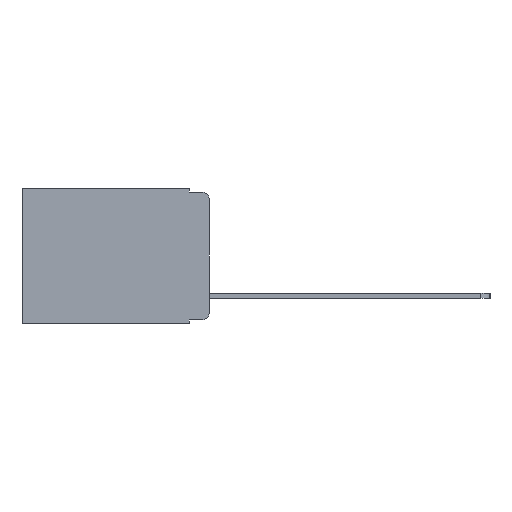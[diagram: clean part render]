
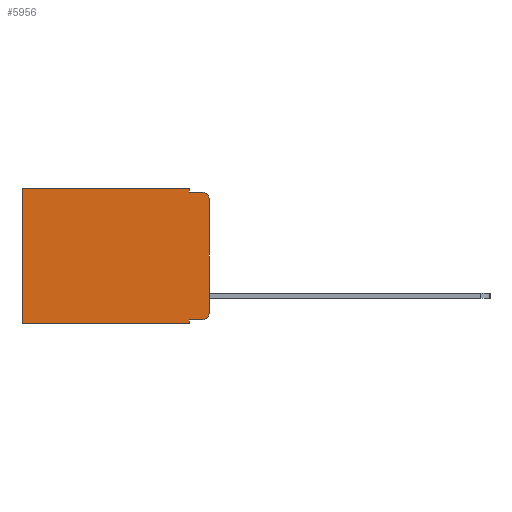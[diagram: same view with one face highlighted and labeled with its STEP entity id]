
A CAD part, left-side view. The second image highlights one B-rep face of the part: STEP entity #5956.
In plain terms, the highlighted planar face has unit normal (-1, 0, 0).
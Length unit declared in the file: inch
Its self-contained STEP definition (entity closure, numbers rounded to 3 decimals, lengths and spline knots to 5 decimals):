
#191 = DIRECTION ( 'NONE',  ( 0., 0., -1. ) ) ;
#523 = CARTESIAN_POINT ( 'NONE',  ( 0.298, 0.051, 0. ) ) ;
#1885 = VERTEX_POINT ( 'NONE', #18534 ) ;
#2325 = VERTEX_POINT ( 'NONE', #20795 ) ;
#2650 = CARTESIAN_POINT ( 'NONE',  ( 0.298, 0.051, -0.01 ) ) ;
#2840 = ORIENTED_EDGE ( 'NONE', *, *, #15150, .T. ) ;
#3032 = DIRECTION ( 'NONE',  ( 0., 1., 0. ) ) ;
#3076 = EDGE_CURVE ( 'NONE', #10299, #19480, #10213, .T. ) ;
#3449 = CARTESIAN_POINT ( 'NONE',  ( 0.298, 0., -0.03 ) ) ;
#4830 = DIRECTION ( 'NONE',  ( 0., 0., -1. ) ) ;
#4920 = EDGE_CURVE ( 'NONE', #17954, #14853, #17145, .T. ) ;
#5129 = VECTOR ( 'NONE', #13450, 39.37008 ) ;
#5503 = AXIS2_PLACEMENT_3D ( 'NONE', #19435, #8144, #21201 ) ;
#5956 = ADVANCED_FACE ( 'NONE', ( #15902 ), #20668, .F. ) ;
#6232 = EDGE_CURVE ( 'NONE', #10166, #14853, #13845, .T. ) ;
#6737 = VECTOR ( 'NONE', #15516, 39.37008 ) ;
#7213 = ORIENTED_EDGE ( 'NONE', *, *, #18138, .F. ) ;
#7403 = ORIENTED_EDGE ( 'NONE', *, *, #11337, .F. ) ;
#7589 = CARTESIAN_POINT ( 'NONE',  ( 0.298, 0., 0. ) ) ;
#7990 = ORIENTED_EDGE ( 'NONE', *, *, #10050, .T. ) ;
#8144 = DIRECTION ( 'NONE',  ( -1., 0., 0. ) ) ;
#8494 = ORIENTED_EDGE ( 'NONE', *, *, #6232, .F. ) ;
#8585 = ORIENTED_EDGE ( 'NONE', *, *, #8775, .F. ) ;
#8637 = CARTESIAN_POINT ( 'NONE',  ( 0.298, 0.473, -0.343 ) ) ;
#8775 = EDGE_CURVE ( 'NONE', #10299, #10166, #18687, .T. ) ;
#9145 = VERTEX_POINT ( 'NONE', #8637 ) ;
#9196 = EDGE_LOOP ( 'NONE', ( #7213, #16076, #8494, #8585, #18636, #7990, #13047, #7403, #2840, #11280 ) ) ;
#9250 = VECTOR ( 'NONE', #4830, 39.37008 ) ;
#9460 = DIRECTION ( 'NONE',  ( 1., 0., 0. ) ) ;
#9505 = CARTESIAN_POINT ( 'NONE',  ( 0.298, 0.02, -0.03 ) ) ;
#9752 = VECTOR ( 'NONE', #20684, 39.37008 ) ;
#10050 = EDGE_CURVE ( 'NONE', #19480, #9145, #14839, .T. ) ;
#10166 = VERTEX_POINT ( 'NONE', #17454 ) ;
#10213 = LINE ( 'NONE', #22612, #5129 ) ;
#10299 = VERTEX_POINT ( 'NONE', #523 ) ;
#10705 = CARTESIAN_POINT ( 'NONE',  ( 0.298, 0., -0.343 ) ) ;
#11264 = AXIS2_PLACEMENT_3D ( 'NONE', #9505, #22533, #11455 ) ;
#11280 = ORIENTED_EDGE ( 'NONE', *, *, #16379, .T. ) ;
#11334 = CARTESIAN_POINT ( 'NONE',  ( 0.298, 0.051, 0. ) ) ;
#11337 = EDGE_CURVE ( 'NONE', #19184, #1885, #24091, .T. ) ;
#11455 = DIRECTION ( 'NONE',  ( 0., 0., -1. ) ) ;
#11761 = CARTESIAN_POINT ( 'NONE',  ( 0.298, 0., 0. ) ) ;
#12386 = LINE ( 'NONE', #13709, #6737 ) ;
#12438 = CARTESIAN_POINT ( 'NONE',  ( 0.298, 0.051, 0. ) ) ;
#12877 = LINE ( 'NONE', #10705, #17303 ) ;
#13047 = ORIENTED_EDGE ( 'NONE', *, *, #17810, .F. ) ;
#13450 = DIRECTION ( 'NONE',  ( 0., 1., 0. ) ) ;
#13705 = VECTOR ( 'NONE', #18805, 39.37008 ) ;
#13709 = CARTESIAN_POINT ( 'NONE',  ( 0.298, 0.051, -0.333 ) ) ;
#13845 = LINE ( 'NONE', #2650, #18266 ) ;
#14839 = LINE ( 'NONE', #17037, #9752 ) ;
#14853 = VERTEX_POINT ( 'NONE', #22093 ) ;
#15150 = EDGE_CURVE ( 'NONE', #19184, #2325, #12386, .T. ) ;
#15516 = DIRECTION ( 'NONE',  ( 0., -1., 0. ) ) ;
#15902 = FACE_OUTER_BOUND ( 'NONE', #9196, .T. ) ;
#16076 = ORIENTED_EDGE ( 'NONE', *, *, #4920, .T. ) ;
#16379 = EDGE_CURVE ( 'NONE', #2325, #23035, #20991, .T. ) ;
#17037 = CARTESIAN_POINT ( 'NONE',  ( 0.298, 0.473, 0. ) ) ;
#17145 = CIRCLE ( 'NONE', #11264, 0.02 ) ;
#17303 = VECTOR ( 'NONE', #3032, 39.37008 ) ;
#17454 = CARTESIAN_POINT ( 'NONE',  ( 0.298, 0.051, -0.01 ) ) ;
#17810 = EDGE_CURVE ( 'NONE', #1885, #9145, #12877, .T. ) ;
#17922 = DIRECTION ( 'NONE',  ( 0., -1., 0. ) ) ;
#17954 = VERTEX_POINT ( 'NONE', #3449 ) ;
#18138 = EDGE_CURVE ( 'NONE', #17954, #23035, #23830, .T. ) ;
#18266 = VECTOR ( 'NONE', #17922, 39.37008 ) ;
#18518 = CARTESIAN_POINT ( 'NONE',  ( 0.298, 0., -0.313 ) ) ;
#18534 = CARTESIAN_POINT ( 'NONE',  ( 0.298, 0.051, -0.343 ) ) ;
#18636 = ORIENTED_EDGE ( 'NONE', *, *, #3076, .T. ) ;
#18687 = LINE ( 'NONE', #11334, #13705 ) ;
#18805 = DIRECTION ( 'NONE',  ( 0., 0., -1. ) ) ;
#19013 = VECTOR ( 'NONE', #191, 39.37008 ) ;
#19184 = VERTEX_POINT ( 'NONE', #20394 ) ;
#19435 = CARTESIAN_POINT ( 'NONE',  ( 0.298, 0.02, -0.313 ) ) ;
#19480 = VERTEX_POINT ( 'NONE', #23084 ) ;
#20394 = CARTESIAN_POINT ( 'NONE',  ( 0.298, 0.051, -0.333 ) ) ;
#20668 = PLANE ( 'NONE',  #21055 ) ;
#20684 = DIRECTION ( 'NONE',  ( 0., 0., -1. ) ) ;
#20795 = CARTESIAN_POINT ( 'NONE',  ( 0.298, 0.02, -0.333 ) ) ;
#20991 = CIRCLE ( 'NONE', #5503, 0.02 ) ;
#21055 = AXIS2_PLACEMENT_3D ( 'NONE', #7589, #9460, #22490 ) ;
#21201 = DIRECTION ( 'NONE',  ( 0., 0., -1. ) ) ;
#22093 = CARTESIAN_POINT ( 'NONE',  ( 0.298, 0.02, -0.01 ) ) ;
#22490 = DIRECTION ( 'NONE',  ( 0., 0., -1. ) ) ;
#22533 = DIRECTION ( 'NONE',  ( -1., 0., 0. ) ) ;
#22612 = CARTESIAN_POINT ( 'NONE',  ( 0.298, 0., 0. ) ) ;
#23035 = VERTEX_POINT ( 'NONE', #18518 ) ;
#23084 = CARTESIAN_POINT ( 'NONE',  ( 0.298, 0.473, 0. ) ) ;
#23830 = LINE ( 'NONE', #11761, #19013 ) ;
#24091 = LINE ( 'NONE', #12438, #9250 ) ;
